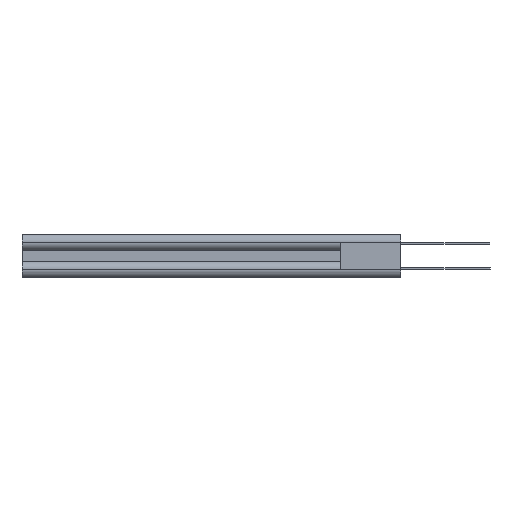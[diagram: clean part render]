
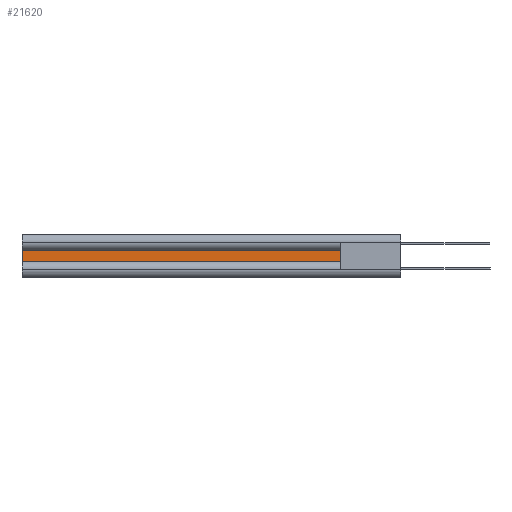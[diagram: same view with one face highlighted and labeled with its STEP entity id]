
A CAD part, left-side view. The second image highlights one B-rep face of the part: STEP entity #21620.
In plain terms, the highlighted planar face has unit normal (-1, 0, 0).
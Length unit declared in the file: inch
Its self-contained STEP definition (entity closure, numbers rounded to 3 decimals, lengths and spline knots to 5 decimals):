
#193 = DIRECTION ( 'NONE',  ( 1., 0., 0. ) ) ;
#336 = CARTESIAN_POINT ( 'NONE',  ( 0.044, 0.473, 0.0465 ) ) ;
#905 = DIRECTION ( 'NONE',  ( 0., 0., -1. ) ) ;
#1460 = AXIS2_PLACEMENT_3D ( 'NONE', #13998, #193, #12357 ) ;
#2671 = EDGE_CURVE ( 'NONE', #17307, #14225, #9540, .T. ) ;
#3335 = DIRECTION ( 'NONE',  ( 0., 0., -1. ) ) ;
#3729 = LINE ( 'NONE', #21093, #16711 ) ;
#3800 = LINE ( 'NONE', #12681, #16792 ) ;
#3870 = VECTOR ( 'NONE', #10025, 39.37008 ) ;
#4743 = ORIENTED_EDGE ( 'NONE', *, *, #21258, .F. ) ;
#5781 = FACE_OUTER_BOUND ( 'NONE', #21793, .T. ) ;
#7761 = ORIENTED_EDGE ( 'NONE', *, *, #13802, .F. ) ;
#8135 = ORIENTED_EDGE ( 'NONE', *, *, #2671, .T. ) ;
#8773 = VECTOR ( 'NONE', #3335, 39.37008 ) ;
#9540 = LINE ( 'NONE', #13513, #3870 ) ;
#9841 = LINE ( 'NONE', #11921, #8773 ) ;
#10025 = DIRECTION ( 'NONE',  ( 0., 1., 0. ) ) ;
#10240 = CARTESIAN_POINT ( 'NONE',  ( 0.044, 0.473, -0.0465 ) ) ;
#11921 = CARTESIAN_POINT ( 'NONE',  ( 0.044, 0.473, -0.0465 ) ) ;
#12357 = DIRECTION ( 'NONE',  ( 0., 0., -1. ) ) ;
#12681 = CARTESIAN_POINT ( 'NONE',  ( 0.044, 0.37012, -0.0465 ) ) ;
#13513 = CARTESIAN_POINT ( 'NONE',  ( 0.044, 0.37012, 0.0465 ) ) ;
#13802 = EDGE_CURVE ( 'NONE', #14147, #18462, #3800, .T. ) ;
#13998 = CARTESIAN_POINT ( 'NONE',  ( 0.044, 0.37012, -0.0465 ) ) ;
#14147 = VERTEX_POINT ( 'NONE', #10240 ) ;
#14225 = VERTEX_POINT ( 'NONE', #21892 ) ;
#14376 = DIRECTION ( 'NONE',  ( 0., 1., 0. ) ) ;
#16711 = VECTOR ( 'NONE', #905, 39.37008 ) ;
#16792 = VECTOR ( 'NONE', #14376, 39.37008 ) ;
#17257 = PLANE ( 'NONE',  #1460 ) ;
#17307 = VERTEX_POINT ( 'NONE', #336 ) ;
#18462 = VERTEX_POINT ( 'NONE', #21883 ) ;
#19380 = EDGE_CURVE ( 'NONE', #14225, #18462, #3729, .T. ) ;
#21093 = CARTESIAN_POINT ( 'NONE',  ( 0.044, 3., -0.0465 ) ) ;
#21258 = EDGE_CURVE ( 'NONE', #17307, #14147, #9841, .T. ) ;
#21620 = ADVANCED_FACE ( 'NONE', ( #5781 ), #17257, .F. ) ;
#21789 = ORIENTED_EDGE ( 'NONE', *, *, #19380, .T. ) ;
#21793 = EDGE_LOOP ( 'NONE', ( #8135, #21789, #7761, #4743 ) ) ;
#21883 = CARTESIAN_POINT ( 'NONE',  ( 0.044, 3., -0.0465 ) ) ;
#21892 = CARTESIAN_POINT ( 'NONE',  ( 0.044, 3., 0.0465 ) ) ;
